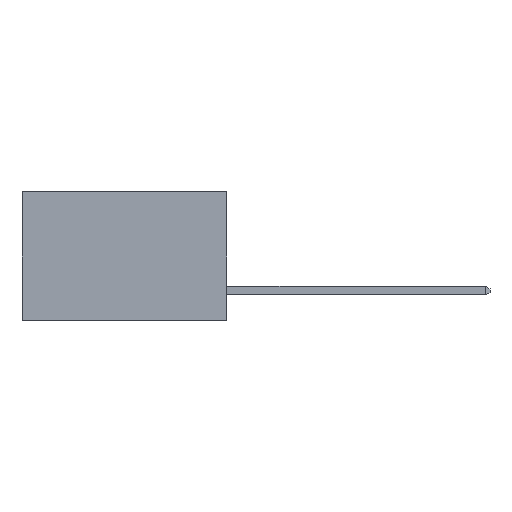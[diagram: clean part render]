
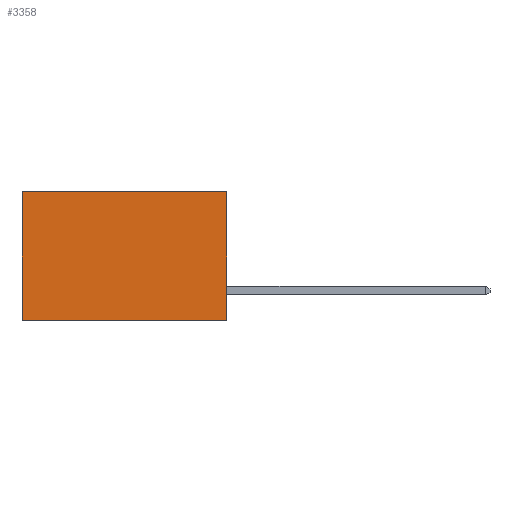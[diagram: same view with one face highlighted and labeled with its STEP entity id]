
A CAD part, left-side view. The second image highlights one B-rep face of the part: STEP entity #3358.
In plain terms, the highlighted planar face has unit normal (-1, 0, 0).
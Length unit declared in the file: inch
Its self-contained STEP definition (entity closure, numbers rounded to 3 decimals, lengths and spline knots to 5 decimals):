
#21 = CARTESIAN_POINT ( 'NONE',  ( 0.277, 0.59, -0.37 ) ) ;
#23 = EDGE_CURVE ( 'NONE', #1831, #4094, #8082, .T. ) ;
#286 = FACE_OUTER_BOUND ( 'NONE', #3144, .T. ) ;
#369 = AXIS2_PLACEMENT_3D ( 'NONE', #3445, #8897, #7565 ) ;
#935 = VERTEX_POINT ( 'NONE', #3563 ) ;
#1065 = VECTOR ( 'NONE', #7368, 39.37008 ) ;
#1239 = ORIENTED_EDGE ( 'NONE', *, *, #23, .T. ) ;
#1241 = LINE ( 'NONE', #10592, #9774 ) ;
#1466 = PLANE ( 'NONE',  #369 ) ;
#1679 = ORIENTED_EDGE ( 'NONE', *, *, #1702, .F. ) ;
#1702 = EDGE_CURVE ( 'NONE', #3626, #4094, #1241, .T. ) ;
#1731 = ORIENTED_EDGE ( 'NONE', *, *, #4936, .F. ) ;
#1741 = ORIENTED_EDGE ( 'NONE', *, *, #6245, .T. ) ;
#1831 = VERTEX_POINT ( 'NONE', #5319 ) ;
#3144 = EDGE_LOOP ( 'NONE', ( #1239, #1679, #1731, #1741 ) ) ;
#3358 = ADVANCED_FACE ( 'NONE', ( #286 ), #1466, .F. ) ;
#3445 = CARTESIAN_POINT ( 'NONE',  ( 0.277, 0., -0.37 ) ) ;
#3563 = CARTESIAN_POINT ( 'NONE',  ( 0.277, 0., 0. ) ) ;
#3626 = VERTEX_POINT ( 'NONE', #10622 ) ;
#4094 = VERTEX_POINT ( 'NONE', #4359 ) ;
#4359 = CARTESIAN_POINT ( 'NONE',  ( 0.277, 0.59, -0.37 ) ) ;
#4936 = EDGE_CURVE ( 'NONE', #935, #3626, #10368, .T. ) ;
#5011 = DIRECTION ( 'NONE',  ( 0., 1., 0. ) ) ;
#5319 = CARTESIAN_POINT ( 'NONE',  ( 0.277, 0.59, 0. ) ) ;
#5451 = CARTESIAN_POINT ( 'NONE',  ( 0.277, 0., 0. ) ) ;
#6057 = VECTOR ( 'NONE', #10224, 39.37008 ) ;
#6245 = EDGE_CURVE ( 'NONE', #935, #1831, #9868, .T. ) ;
#7368 = DIRECTION ( 'NONE',  ( 0., 1., 0. ) ) ;
#7565 = DIRECTION ( 'NONE',  ( 0., 0., -1. ) ) ;
#7816 = VECTOR ( 'NONE', #8808, 39.37008 ) ;
#8082 = LINE ( 'NONE', #21, #7816 ) ;
#8808 = DIRECTION ( 'NONE',  ( 0., 0., -1. ) ) ;
#8897 = DIRECTION ( 'NONE',  ( 1., 0., 0. ) ) ;
#9774 = VECTOR ( 'NONE', #5011, 39.37008 ) ;
#9868 = LINE ( 'NONE', #5451, #1065 ) ;
#10224 = DIRECTION ( 'NONE',  ( 0., 0., -1. ) ) ;
#10368 = LINE ( 'NONE', #10402, #6057 ) ;
#10402 = CARTESIAN_POINT ( 'NONE',  ( 0.277, 0., -0.37 ) ) ;
#10592 = CARTESIAN_POINT ( 'NONE',  ( 0.277, 0., -0.37 ) ) ;
#10622 = CARTESIAN_POINT ( 'NONE',  ( 0.277, 0., -0.37 ) ) ;
